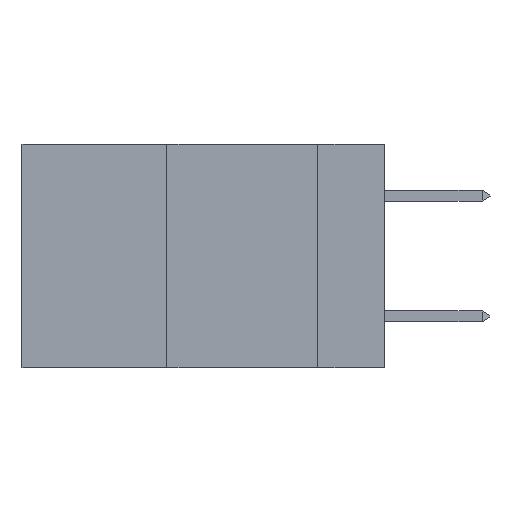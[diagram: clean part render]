
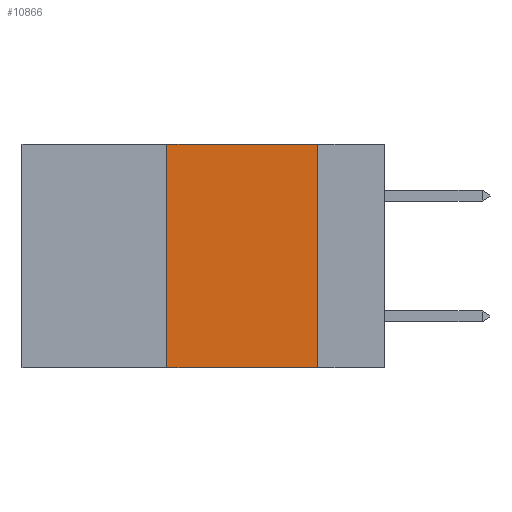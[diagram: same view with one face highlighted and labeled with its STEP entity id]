
A CAD part, left-side view. The second image highlights one B-rep face of the part: STEP entity #10866.
In plain terms, the highlighted planar face has unit normal (-1, 0, 0).
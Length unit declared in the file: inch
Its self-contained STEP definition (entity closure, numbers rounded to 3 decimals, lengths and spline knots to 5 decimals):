
#384 = ORIENTED_EDGE ( 'NONE', *, *, #8963, .F. ) ;
#904 = LINE ( 'NONE', #2103, #10459 ) ;
#1749 = DIRECTION ( 'NONE',  ( 0., -1., 0. ) ) ;
#1917 = ORIENTED_EDGE ( 'NONE', *, *, #6500, .F. ) ;
#2103 = CARTESIAN_POINT ( 'NONE',  ( 0., 0.36, 0. ) ) ;
#2332 = LINE ( 'NONE', #7773, #8497 ) ;
#2920 = VECTOR ( 'NONE', #6527, 39.37008 ) ;
#3430 = CARTESIAN_POINT ( 'NONE',  ( 0., 0.11, -0.37 ) ) ;
#3511 = DIRECTION ( 'NONE',  ( 0., 0., -1. ) ) ;
#4584 = CARTESIAN_POINT ( 'NONE',  ( 0., 0.36, 0. ) ) ;
#4807 = ORIENTED_EDGE ( 'NONE', *, *, #7080, .T. ) ;
#4870 = EDGE_CURVE ( 'NONE', #14107, #8460, #2332, .T. ) ;
#5524 = FACE_OUTER_BOUND ( 'NONE', #7169, .T. ) ;
#5591 = PLANE ( 'NONE',  #12716 ) ;
#6500 = EDGE_CURVE ( 'NONE', #11688, #10954, #904, .T. ) ;
#6527 = DIRECTION ( 'NONE',  ( 0., -1., 0. ) ) ;
#7080 = EDGE_CURVE ( 'NONE', #11688, #8460, #12026, .T. ) ;
#7169 = EDGE_LOOP ( 'NONE', ( #8247, #384, #1917, #4807 ) ) ;
#7515 = CARTESIAN_POINT ( 'NONE',  ( 0., 0.6, 0. ) ) ;
#7773 = CARTESIAN_POINT ( 'NONE',  ( 0., 0.11, 0. ) ) ;
#7920 = CARTESIAN_POINT ( 'NONE',  ( 0., 0.11, 0. ) ) ;
#8247 = ORIENTED_EDGE ( 'NONE', *, *, #4870, .F. ) ;
#8460 = VERTEX_POINT ( 'NONE', #3430 ) ;
#8497 = VECTOR ( 'NONE', #12126, 39.37008 ) ;
#8544 = DIRECTION ( 'NONE',  ( 0., 0., 1. ) ) ;
#8963 = EDGE_CURVE ( 'NONE', #10954, #14107, #12336, .T. ) ;
#10459 = VECTOR ( 'NONE', #8544, 39.37008 ) ;
#10866 = ADVANCED_FACE ( 'NONE', ( #5524 ), #5591, .F. ) ;
#10954 = VERTEX_POINT ( 'NONE', #4584 ) ;
#10966 = CARTESIAN_POINT ( 'NONE',  ( 0., 0.6, -0.37 ) ) ;
#11059 = CARTESIAN_POINT ( 'NONE',  ( 0., 0.36, -0.37 ) ) ;
#11688 = VERTEX_POINT ( 'NONE', #11059 ) ;
#12010 = DIRECTION ( 'NONE',  ( 1., 0., 0. ) ) ;
#12026 = LINE ( 'NONE', #10966, #2920 ) ;
#12126 = DIRECTION ( 'NONE',  ( 0., 0., -1. ) ) ;
#12336 = LINE ( 'NONE', #12487, #13119 ) ;
#12487 = CARTESIAN_POINT ( 'NONE',  ( 0., 0.6, 0. ) ) ;
#12716 = AXIS2_PLACEMENT_3D ( 'NONE', #7515, #12010, #3511 ) ;
#13119 = VECTOR ( 'NONE', #1749, 39.37008 ) ;
#14107 = VERTEX_POINT ( 'NONE', #7920 ) ;
